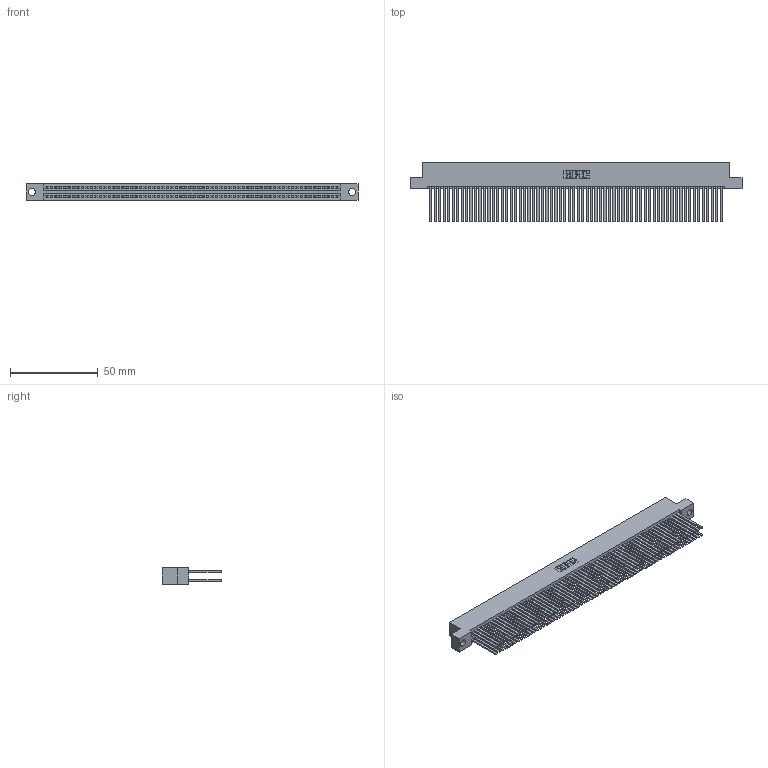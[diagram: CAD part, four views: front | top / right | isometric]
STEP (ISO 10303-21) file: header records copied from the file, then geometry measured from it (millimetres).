
FILE_DESCRIPTION (( 'STEP AP203' ), '1' );
FILE_NAME ('395-132-544-204.STEP', '2021-06-18T01:14:25', ( '' ), ( '' ), 'SwSTEP 2.0', 'SolidWorks 2020', '' );
FILE_SCHEMA (( 'CONFIG_CONTROL_DESIGN' ));
Length unit declared in the file: inch
Products named in the file (3): 395-132-544-204; 345-292-001_345-293-144; 345 Part_Flush Mounting Lugs - 0.156 Dia-TI
Assembly tree (133 placements, depth 2):
  395-132-544-204
    345 Part_Flush Mounting Lugs - 0.156 Dia-TI
    345-292-001_345-293-144  x132
Bounding box: 188.85 x 33.96 x 9.4 mm (x, y, z)
Volume: 20312.2 mm3; surface area: 35764.6 mm2
Topology: 133 solids, 133 shells, 5948 faces, 17669 edges, 11602 vertices
Faces by surface type: plane 3922, cylinder 2026
Entity records: 48789 total; most frequent: CARTESIAN_POINT 8158, ORIENTED_EDGE 8090, DIRECTION 7161, EDGE_CURVE 4045, LINE 3653, VECTOR 3653, VERTEX_POINT 2694, AXIS2_PLACEMENT_3D 1754
